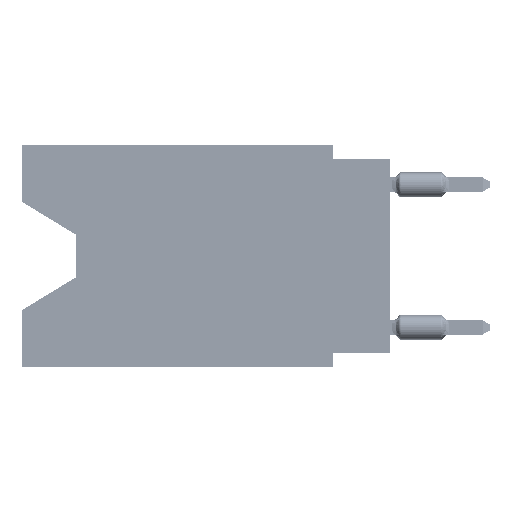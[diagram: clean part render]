
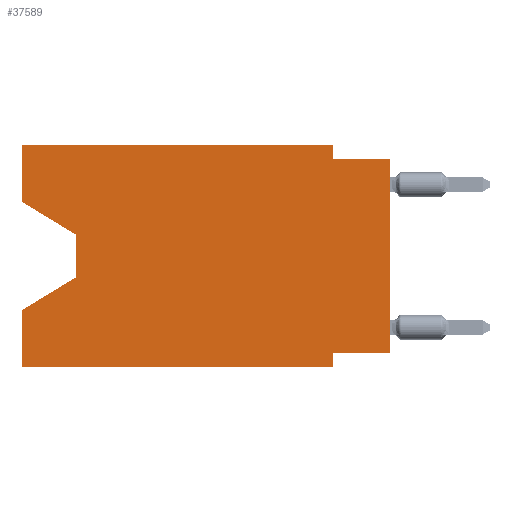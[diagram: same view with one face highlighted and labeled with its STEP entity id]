
A CAD part, left-side view. The second image highlights one B-rep face of the part: STEP entity #37589.
In plain terms, the highlighted planar face has unit normal (-1, 0, 0).
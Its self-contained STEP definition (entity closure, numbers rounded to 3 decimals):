
#851 = VECTOR ( 'NONE', #60241, 1000. ) ;
#1161 = VECTOR ( 'NONE', #73907, 1000. ) ;
#2201 = ORIENTED_EDGE ( 'NONE', *, *, #22808, .T. ) ;
#3306 = CARTESIAN_POINT ( 'NONE',  ( 0., 2.54, -9.906 ) ) ;
#3439 = CARTESIAN_POINT ( 'NONE',  ( 0., 2.54, 0. ) ) ;
#4839 = EDGE_CURVE ( 'NONE', #54134, #19333, #37840, .T. ) ;
#5435 = LINE ( 'NONE', #54976, #25968 ) ;
#5618 = CARTESIAN_POINT ( 'NONE',  ( 0., 13.97, -5.893 ) ) ;
#5940 = CARTESIAN_POINT ( 'NONE',  ( 0., 2.54, -9.271 ) ) ;
#7138 = ORIENTED_EDGE ( 'NONE', *, *, #59832, .F. ) ;
#8327 = CARTESIAN_POINT ( 'NONE',  ( 0., 0., -0.635 ) ) ;
#9584 = ORIENTED_EDGE ( 'NONE', *, *, #26722, .F. ) ;
#9711 = CARTESIAN_POINT ( 'NONE',  ( 0., 2.54, -0.635 ) ) ;
#10304 = ORIENTED_EDGE ( 'NONE', *, *, #35972, .F. ) ;
#12297 = DIRECTION ( 'NONE',  ( 0., -1., 0. ) ) ;
#12491 = DIRECTION ( 'NONE',  ( 0., 0., -1. ) ) ;
#14487 = LINE ( 'NONE', #14892, #63349 ) ;
#14597 = LINE ( 'NONE', #75806, #49486 ) ;
#14892 = CARTESIAN_POINT ( 'NONE',  ( 0., 16.383, -2.546 ) ) ;
#17478 = EDGE_CURVE ( 'NONE', #18776, #54789, #59056, .T. ) ;
#18776 = VERTEX_POINT ( 'NONE', #29839 ) ;
#18996 = CARTESIAN_POINT ( 'NONE',  ( 0., 0., -9.271 ) ) ;
#19221 = VERTEX_POINT ( 'NONE', #46768 ) ;
#19333 = VERTEX_POINT ( 'NONE', #61744 ) ;
#22454 = ORIENTED_EDGE ( 'NONE', *, *, #66157, .T. ) ;
#22608 = LINE ( 'NONE', #41285, #79281 ) ;
#22808 = EDGE_CURVE ( 'NONE', #64303, #54134, #71638, .T. ) ;
#23182 = EDGE_CURVE ( 'NONE', #54789, #63010, #31380, .T. ) ;
#24152 = VERTEX_POINT ( 'NONE', #18996 ) ;
#24694 = DIRECTION ( 'NONE',  ( 1., 0., 0. ) ) ;
#25760 = ORIENTED_EDGE ( 'NONE', *, *, #4839, .T. ) ;
#25968 = VECTOR ( 'NONE', #49313, 1000. ) ;
#26722 = EDGE_CURVE ( 'NONE', #72880, #30042, #14597, .T. ) ;
#26833 = CARTESIAN_POINT ( 'NONE',  ( 0., 16.383, -9.906 ) ) ;
#27106 = DIRECTION ( 'NONE',  ( 0., -0.855, -0.519 ) ) ;
#27677 = VECTOR ( 'NONE', #70991, 1000. ) ;
#27978 = CARTESIAN_POINT ( 'NONE',  ( 0., 0., 0. ) ) ;
#29242 = EDGE_CURVE ( 'NONE', #24152, #63010, #60023, .T. ) ;
#29690 = AXIS2_PLACEMENT_3D ( 'NONE', #75018, #24694, #12491 ) ;
#29839 = CARTESIAN_POINT ( 'NONE',  ( 0., 2.54, 0. ) ) ;
#30042 = VERTEX_POINT ( 'NONE', #3306 ) ;
#31010 = EDGE_CURVE ( 'NONE', #47520, #19333, #46141, .T. ) ;
#31380 = LINE ( 'NONE', #43591, #66631 ) ;
#32072 = CARTESIAN_POINT ( 'NONE',  ( 0., 0., -9.271 ) ) ;
#35972 = EDGE_CURVE ( 'NONE', #24152, #72880, #61729, .T. ) ;
#37589 = ADVANCED_FACE ( 'NONE', ( #63237 ), #67705, .F. ) ;
#37840 = LINE ( 'NONE', #49629, #51637 ) ;
#40833 = CARTESIAN_POINT ( 'NONE',  ( 0., 16.383, 0. ) ) ;
#41285 = CARTESIAN_POINT ( 'NONE',  ( 0., 16.383, 0. ) ) ;
#41943 = VECTOR ( 'NONE', #70471, 1000. ) ;
#43033 = ORIENTED_EDGE ( 'NONE', *, *, #17478, .F. ) ;
#43591 = CARTESIAN_POINT ( 'NONE',  ( 0., 0., -0.635 ) ) ;
#44129 = CARTESIAN_POINT ( 'NONE',  ( 0., 16.383, 0. ) ) ;
#44941 = ORIENTED_EDGE ( 'NONE', *, *, #31010, .F. ) ;
#45176 = ORIENTED_EDGE ( 'NONE', *, *, #23182, .F. ) ;
#46007 = ORIENTED_EDGE ( 'NONE', *, *, #76950, .F. ) ;
#46141 = LINE ( 'NONE', #40833, #41943 ) ;
#46768 = CARTESIAN_POINT ( 'NONE',  ( 0., 16.383, -2.546 ) ) ;
#47520 = VERTEX_POINT ( 'NONE', #26833 ) ;
#49313 = DIRECTION ( 'NONE',  ( 0., -1., 0. ) ) ;
#49486 = VECTOR ( 'NONE', #51046, 1000. ) ;
#49629 = CARTESIAN_POINT ( 'NONE',  ( 0., 13.97, -5.893 ) ) ;
#51046 = DIRECTION ( 'NONE',  ( 0., 0., -1. ) ) ;
#51637 = VECTOR ( 'NONE', #74377, 1000. ) ;
#53070 = DIRECTION ( 'NONE',  ( 0., 0., 1. ) ) ;
#53402 = CARTESIAN_POINT ( 'NONE',  ( 0., 13.97, -4.013 ) ) ;
#54134 = VERTEX_POINT ( 'NONE', #5618 ) ;
#54789 = VERTEX_POINT ( 'NONE', #9711 ) ;
#54976 = CARTESIAN_POINT ( 'NONE',  ( 0., 16.383, 0. ) ) ;
#57217 = EDGE_LOOP ( 'NONE', ( #77992, #2201, #25760, #44941, #22454, #9584, #10304, #79496, #45176, #43033, #46007, #7138 ) ) ;
#59056 = LINE ( 'NONE', #3439, #69799 ) ;
#59832 = EDGE_CURVE ( 'NONE', #19221, #67853, #22608, .T. ) ;
#60023 = LINE ( 'NONE', #27978, #27677 ) ;
#60241 = DIRECTION ( 'NONE',  ( 0., -1., 0. ) ) ;
#61729 = LINE ( 'NONE', #32072, #1161 ) ;
#61744 = CARTESIAN_POINT ( 'NONE',  ( 0., 16.383, -7.36 ) ) ;
#63010 = VERTEX_POINT ( 'NONE', #8327 ) ;
#63237 = FACE_OUTER_BOUND ( 'NONE', #57217, .T. ) ;
#63349 = VECTOR ( 'NONE', #27106, 1000. ) ;
#64303 = VERTEX_POINT ( 'NONE', #53402 ) ;
#66157 = EDGE_CURVE ( 'NONE', #47520, #30042, #78929, .T. ) ;
#66631 = VECTOR ( 'NONE', #12297, 1000. ) ;
#67705 = PLANE ( 'NONE',  #29690 ) ;
#67853 = VERTEX_POINT ( 'NONE', #44129 ) ;
#69799 = VECTOR ( 'NONE', #78551, 1000. ) ;
#70471 = DIRECTION ( 'NONE',  ( 0., 0., 1. ) ) ;
#70991 = DIRECTION ( 'NONE',  ( 0., 0., 1. ) ) ;
#71638 = LINE ( 'NONE', #76246, #78353 ) ;
#72880 = VERTEX_POINT ( 'NONE', #5940 ) ;
#73907 = DIRECTION ( 'NONE',  ( 0., 1., 0. ) ) ;
#74377 = DIRECTION ( 'NONE',  ( 0., 0.855, -0.519 ) ) ;
#75018 = CARTESIAN_POINT ( 'NONE',  ( 0., 16.383, 0. ) ) ;
#75093 = EDGE_CURVE ( 'NONE', #19221, #64303, #14487, .T. ) ;
#75806 = CARTESIAN_POINT ( 'NONE',  ( 0., 2.54, -9.906 ) ) ;
#75843 = DIRECTION ( 'NONE',  ( 0., 0., -1. ) ) ;
#76246 = CARTESIAN_POINT ( 'NONE',  ( 0., 13.97, -4.013 ) ) ;
#76950 = EDGE_CURVE ( 'NONE', #67853, #18776, #5435, .T. ) ;
#77992 = ORIENTED_EDGE ( 'NONE', *, *, #75093, .T. ) ;
#78353 = VECTOR ( 'NONE', #75843, 1000. ) ;
#78551 = DIRECTION ( 'NONE',  ( 0., 0., -1. ) ) ;
#78929 = LINE ( 'NONE', #79717, #851 ) ;
#79281 = VECTOR ( 'NONE', #53070, 1000. ) ;
#79496 = ORIENTED_EDGE ( 'NONE', *, *, #29242, .T. ) ;
#79717 = CARTESIAN_POINT ( 'NONE',  ( 0., 16.383, -9.906 ) ) ;
